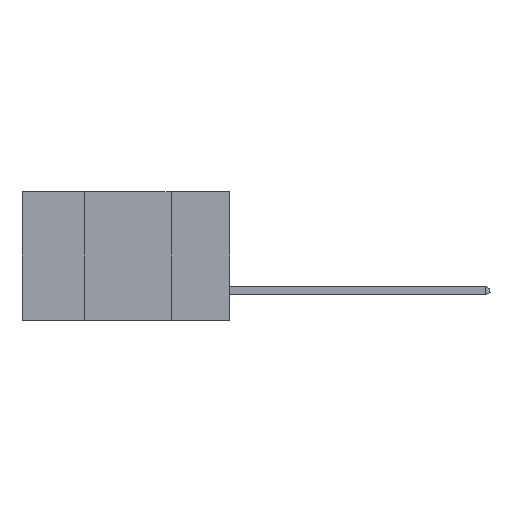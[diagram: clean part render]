
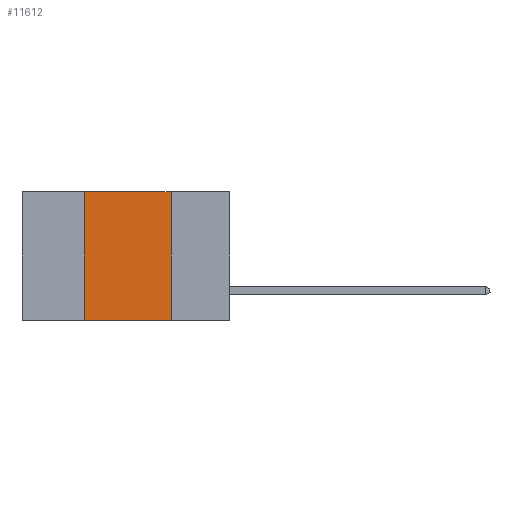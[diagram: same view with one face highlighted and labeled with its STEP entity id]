
A CAD part, left-side view. The second image highlights one B-rep face of the part: STEP entity #11612.
In plain terms, the highlighted planar face has unit normal (-1, 0, 0).
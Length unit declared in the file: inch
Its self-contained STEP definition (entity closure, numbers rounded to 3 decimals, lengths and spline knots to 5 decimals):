
#1300 = LINE ( 'NONE', #6987, #7831 ) ;
#1658 = EDGE_LOOP ( 'NONE', ( #3651, #10662, #6913, #6984 ) ) ;
#1676 = VERTEX_POINT ( 'NONE', #9404 ) ;
#1955 = EDGE_CURVE ( 'NONE', #11775, #11621, #4149, .T. ) ;
#2783 = CARTESIAN_POINT ( 'NONE',  ( 0., 0.6, -0.37 ) ) ;
#3165 = EDGE_CURVE ( 'NONE', #10630, #11775, #3582, .T. ) ;
#3373 = CARTESIAN_POINT ( 'NONE',  ( 0., 0.6, 0. ) ) ;
#3582 = LINE ( 'NONE', #10572, #9590 ) ;
#3651 = ORIENTED_EDGE ( 'NONE', *, *, #1955, .F. ) ;
#4149 = LINE ( 'NONE', #9096, #11678 ) ;
#4453 = DIRECTION ( 'NONE',  ( 0., 0., -1. ) ) ;
#4587 = LINE ( 'NONE', #2783, #10924 ) ;
#4782 = EDGE_CURVE ( 'NONE', #1676, #10630, #1300, .T. ) ;
#5881 = DIRECTION ( 'NONE',  ( 0., 0., 1. ) ) ;
#6279 = EDGE_CURVE ( 'NONE', #1676, #11621, #4587, .T. ) ;
#6371 = DIRECTION ( 'NONE',  ( 0., -1., 0. ) ) ;
#6913 = ORIENTED_EDGE ( 'NONE', *, *, #4782, .F. ) ;
#6951 = DIRECTION ( 'NONE',  ( 0., 0., -1. ) ) ;
#6984 = ORIENTED_EDGE ( 'NONE', *, *, #6279, .T. ) ;
#6987 = CARTESIAN_POINT ( 'NONE',  ( 0., 0.42, 0. ) ) ;
#7831 = VECTOR ( 'NONE', #5881, 39.37008 ) ;
#7844 = FACE_OUTER_BOUND ( 'NONE', #1658, .T. ) ;
#8860 = CARTESIAN_POINT ( 'NONE',  ( 0., 0.17, -0.37 ) ) ;
#9096 = CARTESIAN_POINT ( 'NONE',  ( 0., 0.17, 0. ) ) ;
#9404 = CARTESIAN_POINT ( 'NONE',  ( 0., 0.42, -0.37 ) ) ;
#9590 = VECTOR ( 'NONE', #6371, 39.37008 ) ;
#9964 = DIRECTION ( 'NONE',  ( 1., 0., 0. ) ) ;
#10572 = CARTESIAN_POINT ( 'NONE',  ( 0., 0.6, 0. ) ) ;
#10630 = VERTEX_POINT ( 'NONE', #12664 ) ;
#10662 = ORIENTED_EDGE ( 'NONE', *, *, #3165, .F. ) ;
#10924 = VECTOR ( 'NONE', #12631, 39.37008 ) ;
#11106 = PLANE ( 'NONE',  #12104 ) ;
#11612 = ADVANCED_FACE ( 'NONE', ( #7844 ), #11106, .F. ) ;
#11621 = VERTEX_POINT ( 'NONE', #8860 ) ;
#11678 = VECTOR ( 'NONE', #6951, 39.37008 ) ;
#11775 = VERTEX_POINT ( 'NONE', #12300 ) ;
#12104 = AXIS2_PLACEMENT_3D ( 'NONE', #3373, #9964, #4453 ) ;
#12300 = CARTESIAN_POINT ( 'NONE',  ( 0., 0.17, 0. ) ) ;
#12631 = DIRECTION ( 'NONE',  ( 0., -1., 0. ) ) ;
#12664 = CARTESIAN_POINT ( 'NONE',  ( 0., 0.42, 0. ) ) ;
